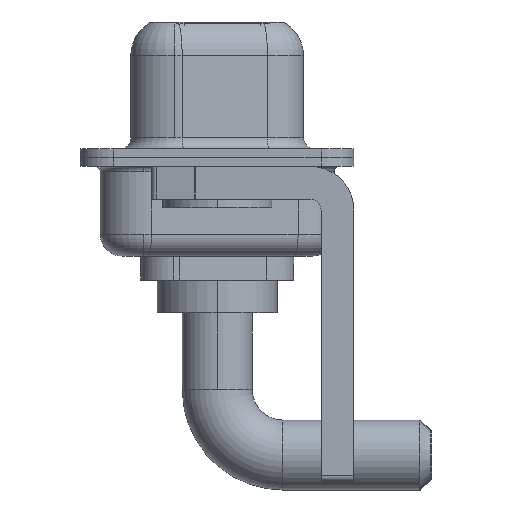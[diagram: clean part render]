
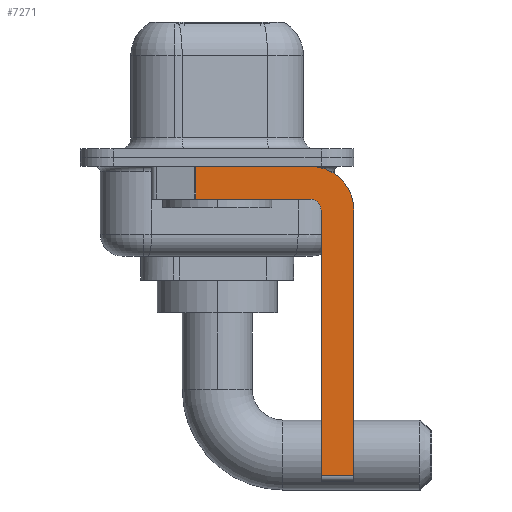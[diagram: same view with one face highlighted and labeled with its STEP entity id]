
A CAD part, left-side view. The second image highlights one B-rep face of the part: STEP entity #7271.
In plain terms, the highlighted planar face has unit normal (-1, 0, 0).
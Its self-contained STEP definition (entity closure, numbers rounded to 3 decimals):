
#141 = EDGE_CURVE ( 'NONE', #8349, #10623, #11686, .T. ) ;
#164 = DIRECTION ( 'NONE',  ( 1., 0., 0. ) ) ;
#325 = ORIENTED_EDGE ( 'NONE', *, *, #2280, .F. ) ;
#639 = CARTESIAN_POINT ( 'NONE',  ( -2.9, 0.978, -1.9 ) ) ;
#681 = ORIENTED_EDGE ( 'NONE', *, *, #1103, .F. ) ;
#948 = CARTESIAN_POINT ( 'NONE',  ( -2.9, -4.25, -2.4 ) ) ;
#1011 = LINE ( 'NONE', #7421, #11943 ) ;
#1103 = EDGE_CURVE ( 'NONE', #10623, #2232, #2745, .T. ) ;
#1729 = ORIENTED_EDGE ( 'NONE', *, *, #6605, .T. ) ;
#1955 = CARTESIAN_POINT ( 'NONE',  ( -2.9, 0.978, -0.4 ) ) ;
#2149 = VECTOR ( 'NONE', #12686, 1000. ) ;
#2232 = VERTEX_POINT ( 'NONE', #2855 ) ;
#2280 = EDGE_CURVE ( 'NONE', #2869, #11374, #1011, .T. ) ;
#2406 = VECTOR ( 'NONE', #3841, 1000. ) ;
#2745 = LINE ( 'NONE', #5671, #9195 ) ;
#2776 = EDGE_CURVE ( 'NONE', #12514, #4354, #8406, .T. ) ;
#2855 = CARTESIAN_POINT ( 'NONE',  ( -2.9, -6.25, -14.55 ) ) ;
#2869 = VERTEX_POINT ( 'NONE', #12032 ) ;
#2912 = DIRECTION ( 'NONE',  ( 0., 0., -1. ) ) ;
#2966 = ORIENTED_EDGE ( 'NONE', *, *, #141, .F. ) ;
#3322 = CARTESIAN_POINT ( 'NONE',  ( -2.9, -4.25, -0.4 ) ) ;
#3504 = AXIS2_PLACEMENT_3D ( 'NONE', #948, #164, #12981 ) ;
#3574 = DIRECTION ( 'NONE',  ( 0., 0., -1. ) ) ;
#3599 = AXIS2_PLACEMENT_3D ( 'NONE', #13900, #5323, #2912 ) ;
#3786 = LINE ( 'NONE', #7064, #10436 ) ;
#3841 = DIRECTION ( 'NONE',  ( 0., -1., 0. ) ) ;
#4034 = EDGE_CURVE ( 'NONE', #10069, #8349, #9268, .T. ) ;
#4052 = FACE_OUTER_BOUND ( 'NONE', #9590, .T. ) ;
#4354 = VERTEX_POINT ( 'NONE', #8827 ) ;
#5323 = DIRECTION ( 'NONE',  ( 1., 0., 0. ) ) ;
#5408 = CIRCLE ( 'NONE', #13855, 0.5 ) ;
#5671 = CARTESIAN_POINT ( 'NONE',  ( -2.9, -6.25, -2.4 ) ) ;
#5706 = LINE ( 'NONE', #13339, #5717 ) ;
#5717 = VECTOR ( 'NONE', #3574, 1000. ) ;
#5993 = DIRECTION ( 'NONE',  ( 0., -1., 0. ) ) ;
#6199 = ORIENTED_EDGE ( 'NONE', *, *, #7754, .F. ) ;
#6353 = CARTESIAN_POINT ( 'NONE',  ( -2.9, -6.25, -2.4 ) ) ;
#6605 = EDGE_CURVE ( 'NONE', #12514, #2232, #3786, .T. ) ;
#6679 = ORIENTED_EDGE ( 'NONE', *, *, #10806, .T. ) ;
#7064 = CARTESIAN_POINT ( 'NONE',  ( -2.9, -4.25, -14.55 ) ) ;
#7271 = ADVANCED_FACE ( 'NONE', ( #4052 ), #9557, .F. ) ;
#7421 = CARTESIAN_POINT ( 'NONE',  ( -2.9, -4.25, -1.9 ) ) ;
#7754 = EDGE_CURVE ( 'NONE', #4354, #2869, #5408, .T. ) ;
#7831 = DIRECTION ( 'NONE',  ( 0., 0., 1. ) ) ;
#8349 = VERTEX_POINT ( 'NONE', #3322 ) ;
#8406 = LINE ( 'NONE', #8550, #2149 ) ;
#8550 = CARTESIAN_POINT ( 'NONE',  ( -2.9, -4.75, -14.8 ) ) ;
#8827 = CARTESIAN_POINT ( 'NONE',  ( -2.9, -4.75, -2.4 ) ) ;
#9195 = VECTOR ( 'NONE', #10031, 1000. ) ;
#9268 = LINE ( 'NONE', #13607, #2406 ) ;
#9557 = PLANE ( 'NONE',  #3599 ) ;
#9590 = EDGE_LOOP ( 'NONE', ( #9845, #6679, #325, #6199, #10014, #1729, #681, #2966 ) ) ;
#9825 = DIRECTION ( 'NONE',  ( -1., 0., 0. ) ) ;
#9845 = ORIENTED_EDGE ( 'NONE', *, *, #4034, .F. ) ;
#10014 = ORIENTED_EDGE ( 'NONE', *, *, #2776, .F. ) ;
#10031 = DIRECTION ( 'NONE',  ( 0., 0., -1. ) ) ;
#10069 = VERTEX_POINT ( 'NONE', #1955 ) ;
#10436 = VECTOR ( 'NONE', #5993, 1000. ) ;
#10623 = VERTEX_POINT ( 'NONE', #6353 ) ;
#10806 = EDGE_CURVE ( 'NONE', #10069, #11374, #5706, .T. ) ;
#11172 = CARTESIAN_POINT ( 'NONE',  ( -2.9, -4.25, -2.4 ) ) ;
#11374 = VERTEX_POINT ( 'NONE', #639 ) ;
#11616 = CARTESIAN_POINT ( 'NONE',  ( -2.9, -4.75, -14.55 ) ) ;
#11686 = CIRCLE ( 'NONE', #3504, 2. ) ;
#11943 = VECTOR ( 'NONE', #12779, 1000. ) ;
#12032 = CARTESIAN_POINT ( 'NONE',  ( -2.9, -4.25, -1.9 ) ) ;
#12514 = VERTEX_POINT ( 'NONE', #11616 ) ;
#12686 = DIRECTION ( 'NONE',  ( 0., 0., 1. ) ) ;
#12779 = DIRECTION ( 'NONE',  ( 0., 1., 0. ) ) ;
#12981 = DIRECTION ( 'NONE',  ( 0., 0., -1. ) ) ;
#13339 = CARTESIAN_POINT ( 'NONE',  ( -2.9, 0.978, -1.9 ) ) ;
#13607 = CARTESIAN_POINT ( 'NONE',  ( -2.9, 3., -0.4 ) ) ;
#13855 = AXIS2_PLACEMENT_3D ( 'NONE', #11172, #9825, #7831 ) ;
#13900 = CARTESIAN_POINT ( 'NONE',  ( -2.9, -4.25, -2.4 ) ) ;
